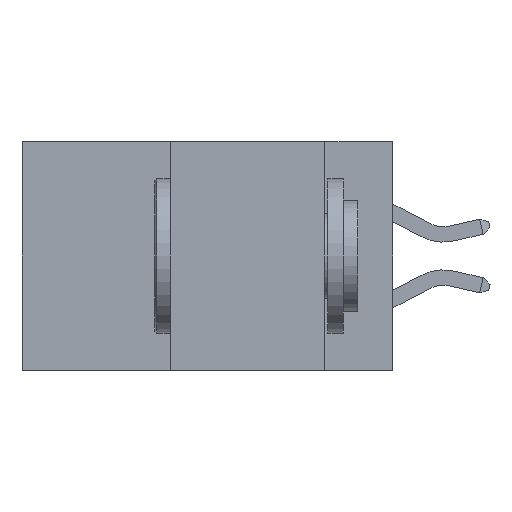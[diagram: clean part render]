
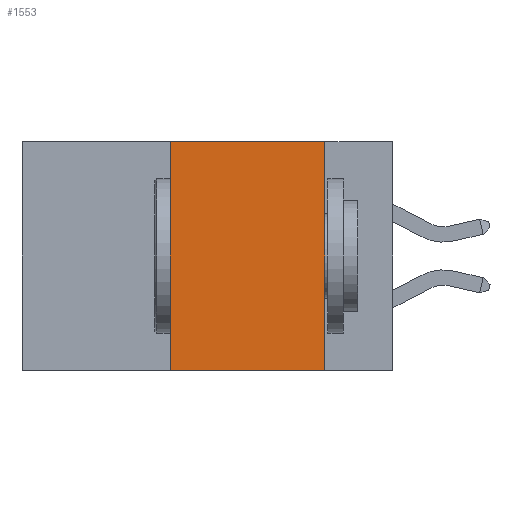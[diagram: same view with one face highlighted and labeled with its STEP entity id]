
A CAD part, left-side view. The second image highlights one B-rep face of the part: STEP entity #1553.
In plain terms, the highlighted planar face has unit normal (-1, 0, 0).
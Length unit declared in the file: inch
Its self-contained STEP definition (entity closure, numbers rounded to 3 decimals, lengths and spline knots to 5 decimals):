
#849 = EDGE_CURVE ( 'NONE', #2288, #2666, #6094, .T. ) ;
#1190 = DIRECTION ( 'NONE',  ( 0., -1., 0. ) ) ;
#1285 = CARTESIAN_POINT ( 'NONE',  ( 0., 0.36, -0.37 ) ) ;
#1553 = ADVANCED_FACE ( 'NONE', ( #14898 ), #4014, .F. ) ;
#1683 = CARTESIAN_POINT ( 'NONE',  ( 0., 0.11, 0. ) ) ;
#1885 = ORIENTED_EDGE ( 'NONE', *, *, #8159, .F. ) ;
#2123 = DIRECTION ( 'NONE',  ( 0., -1., 0. ) ) ;
#2288 = VERTEX_POINT ( 'NONE', #18172 ) ;
#2521 = DIRECTION ( 'NONE',  ( 0., 0., -1. ) ) ;
#2666 = VERTEX_POINT ( 'NONE', #1683 ) ;
#3725 = CARTESIAN_POINT ( 'NONE',  ( 0., 0.6, 0. ) ) ;
#3929 = DIRECTION ( 'NONE',  ( 0., 0., -1. ) ) ;
#4014 = PLANE ( 'NONE',  #18211 ) ;
#4520 = EDGE_LOOP ( 'NONE', ( #1885, #13715, #15665, #13884 ) ) ;
#6094 = LINE ( 'NONE', #22729, #19399 ) ;
#7523 = VECTOR ( 'NONE', #1190, 39.37008 ) ;
#7764 = CARTESIAN_POINT ( 'NONE',  ( 0., 0.11, -0.37 ) ) ;
#8159 = EDGE_CURVE ( 'NONE', #2666, #16066, #16490, .T. ) ;
#8351 = VERTEX_POINT ( 'NONE', #1285 ) ;
#8500 = CARTESIAN_POINT ( 'NONE',  ( 0., 0.36, 0. ) ) ;
#10190 = EDGE_CURVE ( 'NONE', #8351, #2288, #20658, .T. ) ;
#10948 = VECTOR ( 'NONE', #13798, 39.37008 ) ;
#11892 = VECTOR ( 'NONE', #2521, 39.37008 ) ;
#13705 = CARTESIAN_POINT ( 'NONE',  ( 0., 0.6, -0.37 ) ) ;
#13715 = ORIENTED_EDGE ( 'NONE', *, *, #849, .F. ) ;
#13798 = DIRECTION ( 'NONE',  ( 0., 0., 1. ) ) ;
#13884 = ORIENTED_EDGE ( 'NONE', *, *, #19948, .T. ) ;
#14174 = DIRECTION ( 'NONE',  ( 1., 0., 0. ) ) ;
#14898 = FACE_OUTER_BOUND ( 'NONE', #4520, .T. ) ;
#15665 = ORIENTED_EDGE ( 'NONE', *, *, #10190, .F. ) ;
#16066 = VERTEX_POINT ( 'NONE', #7764 ) ;
#16490 = LINE ( 'NONE', #16682, #11892 ) ;
#16682 = CARTESIAN_POINT ( 'NONE',  ( 0., 0.11, 0. ) ) ;
#18172 = CARTESIAN_POINT ( 'NONE',  ( 0., 0.36, 0. ) ) ;
#18211 = AXIS2_PLACEMENT_3D ( 'NONE', #3725, #14174, #3929 ) ;
#19399 = VECTOR ( 'NONE', #2123, 39.37008 ) ;
#19948 = EDGE_CURVE ( 'NONE', #8351, #16066, #21319, .T. ) ;
#20658 = LINE ( 'NONE', #8500, #10948 ) ;
#21319 = LINE ( 'NONE', #13705, #7523 ) ;
#22729 = CARTESIAN_POINT ( 'NONE',  ( 0., 0.6, 0. ) ) ;
